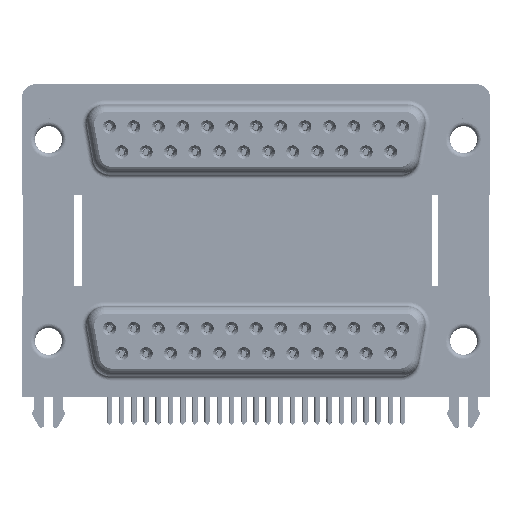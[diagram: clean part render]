
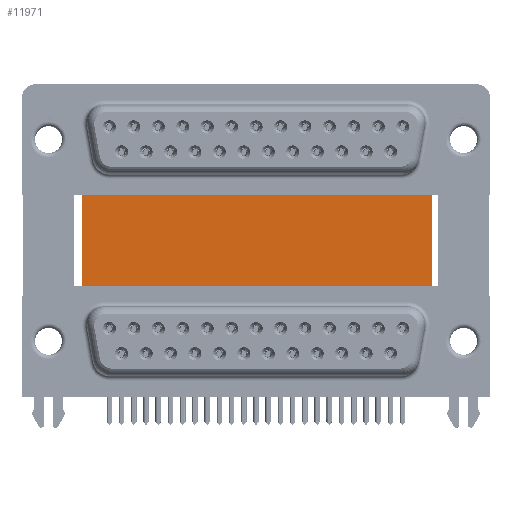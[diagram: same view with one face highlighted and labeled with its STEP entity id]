
A CAD part, top view. The second image highlights one B-rep face of the part: STEP entity #11971.
In plain terms, the highlighted planar face has unit normal (0, 0, 1).
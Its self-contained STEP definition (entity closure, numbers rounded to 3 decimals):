
#302 = VERTEX_POINT ( 'NONE', #8266 ) ;
#2444 = LINE ( 'NONE', #20946, #45055 ) ;
#2866 = VERTEX_POINT ( 'NONE', #20810 ) ;
#6477 = DIRECTION ( 'NONE',  ( -1., 0., 0. ) ) ;
#8266 = CARTESIAN_POINT ( 'NONE',  ( 3.79, -3.735, -12. ) ) ;
#9786 = LINE ( 'NONE', #52494, #13310 ) ;
#9979 = VERTEX_POINT ( 'NONE', #29343 ) ;
#11763 = VECTOR ( 'NONE', #37538, 1000. ) ;
#11917 = CARTESIAN_POINT ( 'NONE',  ( 3.79, -3.735, -12. ) ) ;
#11971 = ADVANCED_FACE ( 'NONE', ( #37998 ), #56500, .F. ) ;
#12318 = EDGE_CURVE ( 'NONE', #2866, #302, #2444, .T. ) ;
#13202 = ORIENTED_EDGE ( 'NONE', *, *, #20389, .F. ) ;
#13310 = VECTOR ( 'NONE', #29467, 1000. ) ;
#14006 = EDGE_CURVE ( 'NONE', #48581, #9979, #9786, .T. ) ;
#14465 = ORIENTED_EDGE ( 'NONE', *, *, #14006, .F. ) ;
#16093 = DIRECTION ( 'NONE',  ( 0., -1., 0. ) ) ;
#20389 = EDGE_CURVE ( 'NONE', #2866, #48581, #46917, .T. ) ;
#20810 = CARTESIAN_POINT ( 'NONE',  ( 3.79, 16.585, -12. ) ) ;
#20946 = CARTESIAN_POINT ( 'NONE',  ( 3.79, 16.585, -12. ) ) ;
#21599 = ORIENTED_EDGE ( 'NONE', *, *, #33968, .T. ) ;
#24210 = CARTESIAN_POINT ( 'NONE',  ( 3.79, 16.585, -12. ) ) ;
#29215 = CARTESIAN_POINT ( 'NONE',  ( 3.79, 16.585, -12. ) ) ;
#29343 = CARTESIAN_POINT ( 'NONE',  ( 43.43, -3.735, -12. ) ) ;
#29359 = ORIENTED_EDGE ( 'NONE', *, *, #12318, .T. ) ;
#29467 = DIRECTION ( 'NONE',  ( 0., -1., 0. ) ) ;
#33968 = EDGE_CURVE ( 'NONE', #302, #9979, #34952, .T. ) ;
#34265 = EDGE_LOOP ( 'NONE', ( #21599, #14465, #13202, #29359 ) ) ;
#34952 = LINE ( 'NONE', #11917, #57798 ) ;
#36661 = CARTESIAN_POINT ( 'NONE',  ( 43.43, 16.585, -12. ) ) ;
#37538 = DIRECTION ( 'NONE',  ( 1., 0., 0. ) ) ;
#37998 = FACE_OUTER_BOUND ( 'NONE', #34265, .T. ) ;
#43058 = AXIS2_PLACEMENT_3D ( 'NONE', #29215, #47690, #6477 ) ;
#44631 = DIRECTION ( 'NONE',  ( 1., 0., 0. ) ) ;
#45055 = VECTOR ( 'NONE', #16093, 1000. ) ;
#46917 = LINE ( 'NONE', #24210, #11763 ) ;
#47690 = DIRECTION ( 'NONE',  ( 0., 0., -1. ) ) ;
#48581 = VERTEX_POINT ( 'NONE', #36661 ) ;
#52494 = CARTESIAN_POINT ( 'NONE',  ( 43.43, 16.585, -12. ) ) ;
#56500 = PLANE ( 'NONE',  #43058 ) ;
#57798 = VECTOR ( 'NONE', #44631, 1000. ) ;
